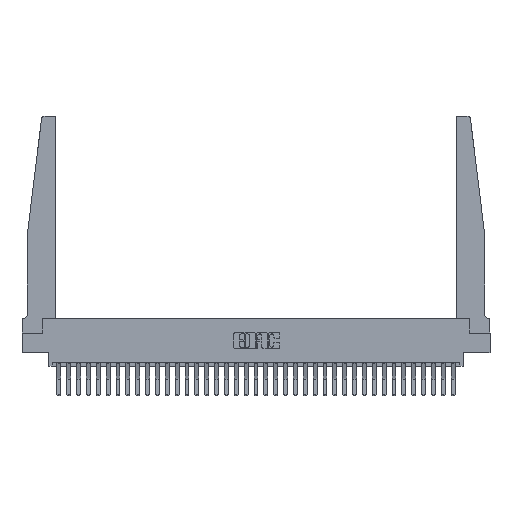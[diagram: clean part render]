
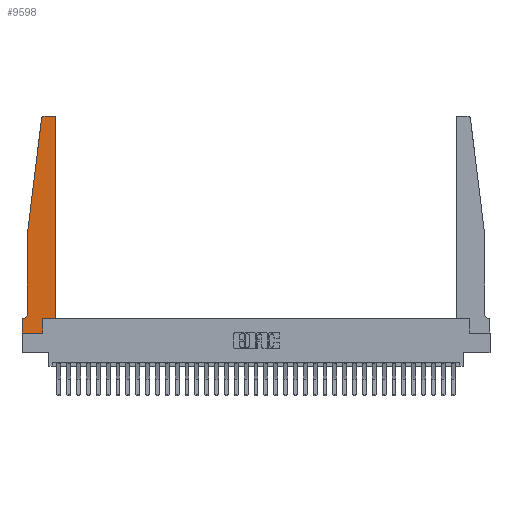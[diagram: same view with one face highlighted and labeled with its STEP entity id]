
A CAD part, top view. The second image highlights one B-rep face of the part: STEP entity #9598.
In plain terms, the highlighted planar face has unit normal (0, 0, 1).
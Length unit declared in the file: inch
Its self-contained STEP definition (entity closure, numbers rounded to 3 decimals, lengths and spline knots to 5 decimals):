
#268 = CARTESIAN_POINT ( 'NONE',  ( 0.2605, 0.18, 0.37 ) ) ;
#706 = ORIENTED_EDGE ( 'NONE', *, *, #2471, .T. ) ;
#910 = VECTOR ( 'NONE', #5232, 39.37008 ) ;
#1275 = AXIS2_PLACEMENT_3D ( 'NONE', #6780, #24080, #9277 ) ;
#1689 = VECTOR ( 'NONE', #31311, 39.37008 ) ;
#1786 = DIRECTION ( 'NONE',  ( -1., 0., 0. ) ) ;
#2035 = EDGE_CURVE ( 'NONE', #12568, #23123, #3806, .T. ) ;
#2059 = CARTESIAN_POINT ( 'NONE',  ( 0., 0.1875, 0.37 ) ) ;
#2222 = DIRECTION ( 'NONE',  ( 1., 0., 0. ) ) ;
#2361 = VECTOR ( 'NONE', #1786, 39.37008 ) ;
#2452 = CARTESIAN_POINT ( 'NONE',  ( 0.25, 2.75, 0.37 ) ) ;
#2471 = EDGE_CURVE ( 'NONE', #11871, #24464, #31194, .T. ) ;
#2637 = VERTEX_POINT ( 'NONE', #3498 ) ;
#2654 = CARTESIAN_POINT ( 'NONE',  ( 0.395, 2.72, 0.37 ) ) ;
#3074 = CARTESIAN_POINT ( 'NONE',  ( 0.24675, 2.72367, 0.37 ) ) ;
#3498 = CARTESIAN_POINT ( 'NONE',  ( 0., 0., 0.37 ) ) ;
#3566 = EDGE_LOOP ( 'NONE', ( #706, #27616, #27932, #14632, #25456, #26456, #30490, #31844, #10351, #20202, #25143, #14417 ) ) ;
#3610 = FACE_OUTER_BOUND ( 'NONE', #3566, .T. ) ;
#3619 = VERTEX_POINT ( 'NONE', #2059 ) ;
#3764 = CARTESIAN_POINT ( 'NONE',  ( 0.065, 0.2375, 0.37 ) ) ;
#3777 = LINE ( 'NONE', #7050, #27721 ) ;
#3806 = LINE ( 'NONE', #13137, #23521 ) ;
#3867 = VECTOR ( 'NONE', #31244, 39.37008 ) ;
#4234 = VECTOR ( 'NONE', #10003, 39.37008 ) ;
#4924 = VERTEX_POINT ( 'NONE', #14719 ) ;
#5124 = DIRECTION ( 'NONE',  ( 1., 0., 0. ) ) ;
#5232 = DIRECTION ( 'NONE',  ( 1., 0., 0. ) ) ;
#5510 = PLANE ( 'NONE',  #26916 ) ;
#5855 = CARTESIAN_POINT ( 'NONE',  ( 0.27653, 2.75, 0.37 ) ) ;
#6198 = EDGE_CURVE ( 'NONE', #2637, #11063, #20611, .T. ) ;
#6780 = CARTESIAN_POINT ( 'NONE',  ( 0.015, 0.2375, 0.37 ) ) ;
#6820 = DIRECTION ( 'NONE',  ( 0., 0., 1. ) ) ;
#7050 = CARTESIAN_POINT ( 'NONE',  ( 0.425, 0.18, 0.37 ) ) ;
#7354 = EDGE_CURVE ( 'NONE', #24464, #10849, #9302, .T. ) ;
#7715 = CARTESIAN_POINT ( 'NONE',  ( 0., 0., 0.37 ) ) ;
#7990 = DIRECTION ( 'NONE',  ( 0., 0., 1. ) ) ;
#8016 = EDGE_CURVE ( 'NONE', #23123, #4924, #13358, .T. ) ;
#9123 = DIRECTION ( 'NONE',  ( -0.122, -0.992, 0. ) ) ;
#9277 = DIRECTION ( 'NONE',  ( -1., 0., 0. ) ) ;
#9302 = CIRCLE ( 'NONE', #31216, 0.03 ) ;
#9598 = ADVANCED_FACE ( 'NONE', ( #3610 ), #5510, .T. ) ;
#9914 = EDGE_CURVE ( 'NONE', #3619, #2637, #27174, .T. ) ;
#10003 = DIRECTION ( 'NONE',  ( 0., 1., 0. ) ) ;
#10351 = ORIENTED_EDGE ( 'NONE', *, *, #29306, .T. ) ;
#10849 = VERTEX_POINT ( 'NONE', #3074 ) ;
#10994 = VECTOR ( 'NONE', #9123, 39.37008 ) ;
#11054 = EDGE_CURVE ( 'NONE', #4924, #3619, #28626, .T. ) ;
#11063 = VERTEX_POINT ( 'NONE', #31442 ) ;
#11220 = LINE ( 'NONE', #11490, #3867 ) ;
#11490 = CARTESIAN_POINT ( 'NONE',  ( 0.425, 0.18, 0.37 ) ) ;
#11587 = LINE ( 'NONE', #22315, #4234 ) ;
#11871 = VERTEX_POINT ( 'NONE', #15560 ) ;
#12417 = EDGE_CURVE ( 'NONE', #29367, #11871, #13120, .T. ) ;
#12568 = VERTEX_POINT ( 'NONE', #30176 ) ;
#13120 = CIRCLE ( 'NONE', #18960, 0.03 ) ;
#13137 = CARTESIAN_POINT ( 'NONE',  ( 0.065, 1.25, 0.37 ) ) ;
#13358 = CIRCLE ( 'NONE', #1275, 0.05 ) ;
#14035 = CARTESIAN_POINT ( 'NONE',  ( 0., 0., 0.37 ) ) ;
#14417 = ORIENTED_EDGE ( 'NONE', *, *, #12417, .T. ) ;
#14632 = ORIENTED_EDGE ( 'NONE', *, *, #2035, .T. ) ;
#14719 = CARTESIAN_POINT ( 'NONE',  ( 0.015, 0.1875, 0.37 ) ) ;
#15091 = CARTESIAN_POINT ( 'NONE',  ( 0.425, 2.72, 0.37 ) ) ;
#15560 = CARTESIAN_POINT ( 'NONE',  ( 0.395, 2.75, 0.37 ) ) ;
#17458 = CARTESIAN_POINT ( 'NONE',  ( 0.425, 0.18, 0.37 ) ) ;
#18123 = DIRECTION ( 'NONE',  ( 0., -1., 0. ) ) ;
#18217 = VERTEX_POINT ( 'NONE', #17458 ) ;
#18960 = AXIS2_PLACEMENT_3D ( 'NONE', #2654, #19926, #5124 ) ;
#19047 = EDGE_CURVE ( 'NONE', #31592, #18217, #3777, .T. ) ;
#19707 = DIRECTION ( 'NONE',  ( -1., 0., 0. ) ) ;
#19926 = DIRECTION ( 'NONE',  ( 0., 0., 1. ) ) ;
#20202 = ORIENTED_EDGE ( 'NONE', *, *, #19047, .T. ) ;
#20611 = LINE ( 'NONE', #7715, #910 ) ;
#20865 = EDGE_CURVE ( 'NONE', #10849, #12568, #25709, .T. ) ;
#21449 = CARTESIAN_POINT ( 'NONE',  ( 0.065, 1.25, 0.37 ) ) ;
#21633 = CARTESIAN_POINT ( 'NONE',  ( 0.27653, 2.72, 0.37 ) ) ;
#22315 = CARTESIAN_POINT ( 'NONE',  ( 0.2605, 0.18, 0.37 ) ) ;
#23123 = VERTEX_POINT ( 'NONE', #3764 ) ;
#23521 = VECTOR ( 'NONE', #18123, 39.37008 ) ;
#23867 = VECTOR ( 'NONE', #19707, 39.37008 ) ;
#24022 = CARTESIAN_POINT ( 'NONE',  ( 0.065, 0.1875, 0.37 ) ) ;
#24080 = DIRECTION ( 'NONE',  ( 0., 0., -1. ) ) ;
#24115 = DIRECTION ( 'NONE',  ( 1., 0., 0. ) ) ;
#24464 = VERTEX_POINT ( 'NONE', #5855 ) ;
#25143 = ORIENTED_EDGE ( 'NONE', *, *, #26247, .T. ) ;
#25300 = DIRECTION ( 'NONE',  ( 1., 0., 0. ) ) ;
#25456 = ORIENTED_EDGE ( 'NONE', *, *, #8016, .T. ) ;
#25709 = LINE ( 'NONE', #21449, #10994 ) ;
#26247 = EDGE_CURVE ( 'NONE', #18217, #29367, #11220, .T. ) ;
#26456 = ORIENTED_EDGE ( 'NONE', *, *, #11054, .T. ) ;
#26916 = AXIS2_PLACEMENT_3D ( 'NONE', #30127, #7990, #25300 ) ;
#27174 = LINE ( 'NONE', #14035, #1689 ) ;
#27616 = ORIENTED_EDGE ( 'NONE', *, *, #7354, .T. ) ;
#27721 = VECTOR ( 'NONE', #2222, 39.37008 ) ;
#27932 = ORIENTED_EDGE ( 'NONE', *, *, #20865, .T. ) ;
#28626 = LINE ( 'NONE', #24022, #2361 ) ;
#29306 = EDGE_CURVE ( 'NONE', #11063, #31592, #11587, .T. ) ;
#29367 = VERTEX_POINT ( 'NONE', #15091 ) ;
#30127 = CARTESIAN_POINT ( 'NONE',  ( 0., 0.1875, 0.37 ) ) ;
#30176 = CARTESIAN_POINT ( 'NONE',  ( 0.065, 1.25, 0.37 ) ) ;
#30490 = ORIENTED_EDGE ( 'NONE', *, *, #9914, .T. ) ;
#31194 = LINE ( 'NONE', #2452, #23867 ) ;
#31216 = AXIS2_PLACEMENT_3D ( 'NONE', #21633, #6820, #24115 ) ;
#31244 = DIRECTION ( 'NONE',  ( 0., 1., 0. ) ) ;
#31311 = DIRECTION ( 'NONE',  ( 0., -1., 0. ) ) ;
#31442 = CARTESIAN_POINT ( 'NONE',  ( 0.2605, 0., 0.37 ) ) ;
#31592 = VERTEX_POINT ( 'NONE', #268 ) ;
#31844 = ORIENTED_EDGE ( 'NONE', *, *, #6198, .T. ) ;
